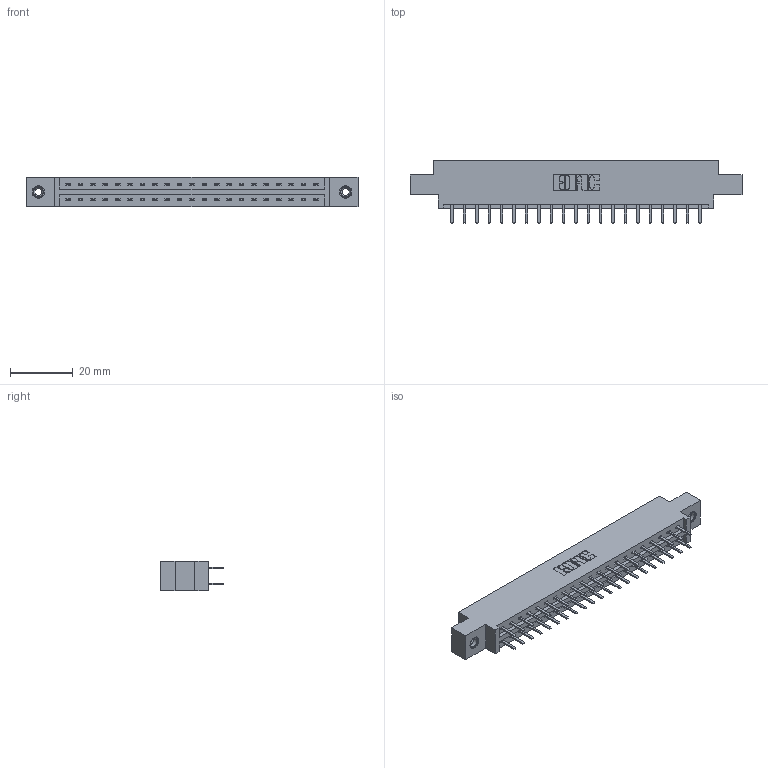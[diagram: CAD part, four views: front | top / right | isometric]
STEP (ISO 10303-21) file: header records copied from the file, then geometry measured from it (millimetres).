
FILE_DESCRIPTION (( 'STEP AP203' ), '1' );
FILE_NAME ('337-042-520-808.STEP', '2018-08-08T23:09:10', ( '' ), ( '' ), 'SwSTEP 2.0', 'SolidWorks 2016', '' );
FILE_SCHEMA (( 'CONFIG_CONTROL_DESIGN' ));
Length unit declared in the file: inch
Products named in the file (4): 345-292-001_345-293-120; 345-250-001_345-250-003-102; 337-042-520-808; 337 Part_0.170 Offset - 0.156 Dia-TI
Assembly tree (45 placements, depth 2):
  337-042-520-808
    337 Part_0.170 Offset - 0.156 Dia-TI
    345-292-001_345-293-120  x42
    345-250-001_345-250-003-102  x2
Bounding box: 106.22 x 20.02 x 9.4 mm (x, y, z)
Volume: 10772.6 mm3; surface area: 12053.5 mm2
Topology: 45 solids, 45 shells, 2614 faces, 7557 edges, 4918 vertices
Faces by surface type: plane 1786, cylinder 812, cone 12, torus 4
Entity records: 20430 total; most frequent: CARTESIAN_POINT 3453, ORIENTED_EDGE 3370, DIRECTION 2995, EDGE_CURVE 1685, LINE 1533, VECTOR 1533, VERTEX_POINT 1116, AXIS2_PLACEMENT_3D 731
